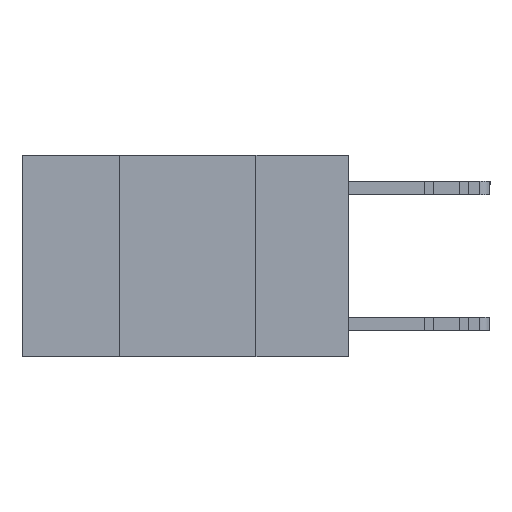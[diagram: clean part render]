
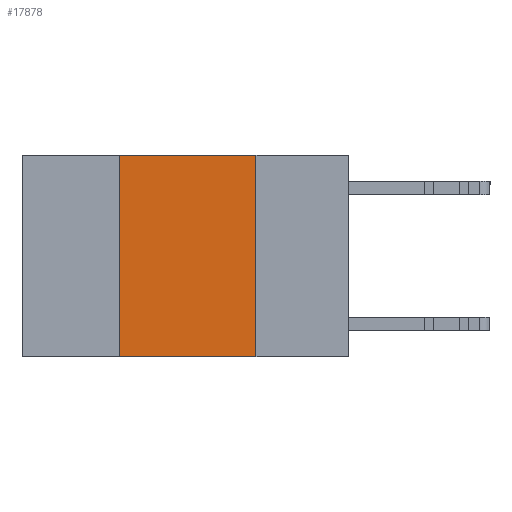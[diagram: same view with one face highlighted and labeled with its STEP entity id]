
A CAD part, left-side view. The second image highlights one B-rep face of the part: STEP entity #17878.
In plain terms, the highlighted planar face has unit normal (-1, 0, 0).
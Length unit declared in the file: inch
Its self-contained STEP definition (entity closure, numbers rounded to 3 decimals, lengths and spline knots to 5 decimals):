
#1375 = CARTESIAN_POINT ( 'NONE',  ( 0., 0.6, 0. ) ) ;
#1439 = CARTESIAN_POINT ( 'NONE',  ( 0., 0.17, 0. ) ) ;
#1530 = ORIENTED_EDGE ( 'NONE', *, *, #17949, .F. ) ;
#2875 = VECTOR ( 'NONE', #9354, 39.37008 ) ;
#3301 = PLANE ( 'NONE',  #12073 ) ;
#6032 = EDGE_CURVE ( 'NONE', #14726, #6224, #10682, .T. ) ;
#6224 = VERTEX_POINT ( 'NONE', #16226 ) ;
#6358 = VECTOR ( 'NONE', #11949, 39.37008 ) ;
#8145 = VECTOR ( 'NONE', #8583, 39.37008 ) ;
#8270 = DIRECTION ( 'NONE',  ( 0., 0., -1. ) ) ;
#8583 = DIRECTION ( 'NONE',  ( 0., 0., -1. ) ) ;
#9101 = EDGE_CURVE ( 'NONE', #29229, #14726, #16609, .T. ) ;
#9354 = DIRECTION ( 'NONE',  ( 0., -1., 0. ) ) ;
#9653 = CARTESIAN_POINT ( 'NONE',  ( 0., 0.6, -0.37 ) ) ;
#10592 = CARTESIAN_POINT ( 'NONE',  ( 0., 0.6, 0. ) ) ;
#10682 = LINE ( 'NONE', #1375, #12211 ) ;
#11949 = DIRECTION ( 'NONE',  ( 0., 0., 1. ) ) ;
#12073 = AXIS2_PLACEMENT_3D ( 'NONE', #10592, #20047, #8270 ) ;
#12211 = VECTOR ( 'NONE', #20299, 39.37008 ) ;
#12897 = CARTESIAN_POINT ( 'NONE',  ( 0., 0.42, 0. ) ) ;
#14726 = VERTEX_POINT ( 'NONE', #12897 ) ;
#15347 = CARTESIAN_POINT ( 'NONE',  ( 0., 0.42, -0.37 ) ) ;
#16226 = CARTESIAN_POINT ( 'NONE',  ( 0., 0.17, 0. ) ) ;
#16609 = LINE ( 'NONE', #30567, #6358 ) ;
#17663 = ORIENTED_EDGE ( 'NONE', *, *, #6032, .F. ) ;
#17878 = ADVANCED_FACE ( 'NONE', ( #24537 ), #3301, .F. ) ;
#17949 = EDGE_CURVE ( 'NONE', #6224, #25823, #29807, .T. ) ;
#20047 = DIRECTION ( 'NONE',  ( 1., 0., 0. ) ) ;
#20299 = DIRECTION ( 'NONE',  ( 0., -1., 0. ) ) ;
#21925 = EDGE_LOOP ( 'NONE', ( #1530, #17663, #25867, #26066 ) ) ;
#24088 = EDGE_CURVE ( 'NONE', #29229, #25823, #25160, .T. ) ;
#24537 = FACE_OUTER_BOUND ( 'NONE', #21925, .T. ) ;
#25160 = LINE ( 'NONE', #9653, #2875 ) ;
#25823 = VERTEX_POINT ( 'NONE', #30540 ) ;
#25867 = ORIENTED_EDGE ( 'NONE', *, *, #9101, .F. ) ;
#26066 = ORIENTED_EDGE ( 'NONE', *, *, #24088, .T. ) ;
#29229 = VERTEX_POINT ( 'NONE', #15347 ) ;
#29807 = LINE ( 'NONE', #1439, #8145 ) ;
#30540 = CARTESIAN_POINT ( 'NONE',  ( 0., 0.17, -0.37 ) ) ;
#30567 = CARTESIAN_POINT ( 'NONE',  ( 0., 0.42, 0. ) ) ;
